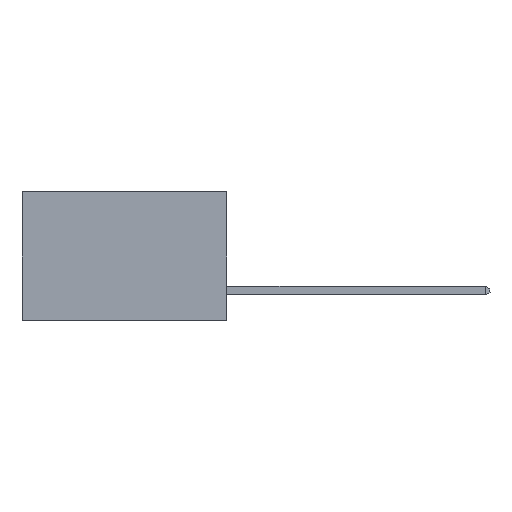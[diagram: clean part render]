
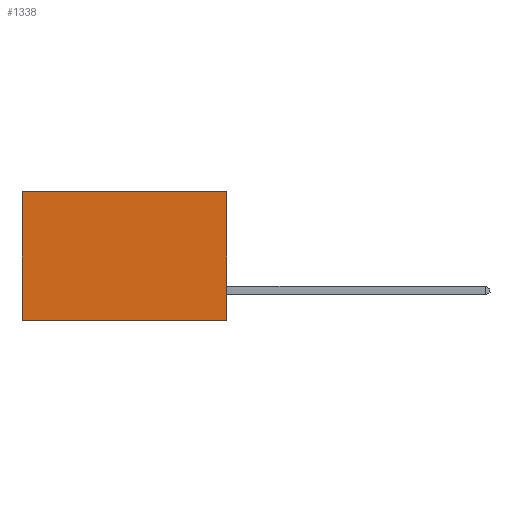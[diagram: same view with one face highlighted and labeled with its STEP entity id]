
A CAD part, left-side view. The second image highlights one B-rep face of the part: STEP entity #1338.
In plain terms, the highlighted planar face has unit normal (-1, 0, 0).
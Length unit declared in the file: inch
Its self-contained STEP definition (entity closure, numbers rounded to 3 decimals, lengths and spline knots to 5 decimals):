
#144 = FACE_OUTER_BOUND ( 'NONE', #1271, .T. ) ;
#170 = CARTESIAN_POINT ( 'NONE',  ( 0.277, 0.59, -0.37 ) ) ;
#205 = DIRECTION ( 'NONE',  ( 0., 0., -1. ) ) ;
#306 = DIRECTION ( 'NONE',  ( 0., 1., 0. ) ) ;
#735 = EDGE_CURVE ( 'NONE', #2390, #3871, #1765, .T. ) ;
#907 = ORIENTED_EDGE ( 'NONE', *, *, #6963, .T. ) ;
#1039 = DIRECTION ( 'NONE',  ( 0., 0., -1. ) ) ;
#1215 = PLANE ( 'NONE',  #4035 ) ;
#1271 = EDGE_LOOP ( 'NONE', ( #907, #2294, #3247, #1677 ) ) ;
#1338 = ADVANCED_FACE ( 'NONE', ( #144 ), #1215, .F. ) ;
#1677 = ORIENTED_EDGE ( 'NONE', *, *, #7087, .T. ) ;
#1765 = LINE ( 'NONE', #6156, #3740 ) ;
#1837 = LINE ( 'NONE', #170, #6962 ) ;
#2294 = ORIENTED_EDGE ( 'NONE', *, *, #6070, .F. ) ;
#2390 = VERTEX_POINT ( 'NONE', #6999 ) ;
#2634 = CARTESIAN_POINT ( 'NONE',  ( 0.277, 0., 0. ) ) ;
#2942 = LINE ( 'NONE', #4693, #7865 ) ;
#3211 = VERTEX_POINT ( 'NONE', #8345 ) ;
#3247 = ORIENTED_EDGE ( 'NONE', *, *, #735, .F. ) ;
#3740 = VECTOR ( 'NONE', #1039, 39.37008 ) ;
#3871 = VERTEX_POINT ( 'NONE', #7564 ) ;
#4022 = DIRECTION ( 'NONE',  ( 0., 1., 0. ) ) ;
#4035 = AXIS2_PLACEMENT_3D ( 'NONE', #4883, #8278, #4626 ) ;
#4626 = DIRECTION ( 'NONE',  ( 0., 0., -1. ) ) ;
#4693 = CARTESIAN_POINT ( 'NONE',  ( 0.277, 0., -0.37 ) ) ;
#4883 = CARTESIAN_POINT ( 'NONE',  ( 0.277, 0., -0.37 ) ) ;
#6070 = EDGE_CURVE ( 'NONE', #3871, #3211, #2942, .T. ) ;
#6128 = VECTOR ( 'NONE', #306, 39.37008 ) ;
#6156 = CARTESIAN_POINT ( 'NONE',  ( 0.277, 0., -0.37 ) ) ;
#6342 = CARTESIAN_POINT ( 'NONE',  ( 0.277, 0.59, 0. ) ) ;
#6344 = LINE ( 'NONE', #2634, #6128 ) ;
#6962 = VECTOR ( 'NONE', #205, 39.37008 ) ;
#6963 = EDGE_CURVE ( 'NONE', #7388, #3211, #1837, .T. ) ;
#6999 = CARTESIAN_POINT ( 'NONE',  ( 0.277, 0., 0. ) ) ;
#7087 = EDGE_CURVE ( 'NONE', #2390, #7388, #6344, .T. ) ;
#7388 = VERTEX_POINT ( 'NONE', #6342 ) ;
#7564 = CARTESIAN_POINT ( 'NONE',  ( 0.277, 0., -0.37 ) ) ;
#7865 = VECTOR ( 'NONE', #4022, 39.37008 ) ;
#8278 = DIRECTION ( 'NONE',  ( 1., 0., 0. ) ) ;
#8345 = CARTESIAN_POINT ( 'NONE',  ( 0.277, 0.59, -0.37 ) ) ;
